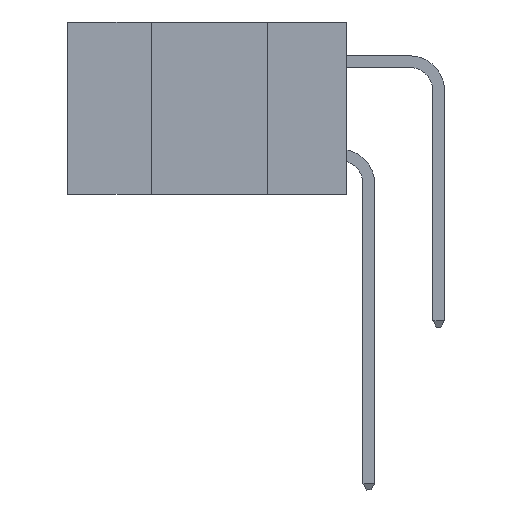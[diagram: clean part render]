
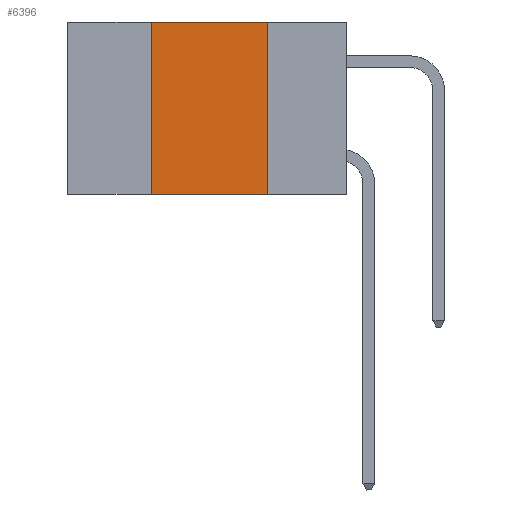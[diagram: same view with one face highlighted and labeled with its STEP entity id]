
A CAD part, left-side view. The second image highlights one B-rep face of the part: STEP entity #6396.
In plain terms, the highlighted planar face has unit normal (-1, 0, 0).
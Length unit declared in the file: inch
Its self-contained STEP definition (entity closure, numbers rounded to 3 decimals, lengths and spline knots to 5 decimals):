
#652 = CARTESIAN_POINT ( 'NONE',  ( 0., 0.6, 0. ) ) ;
#796 = FACE_OUTER_BOUND ( 'NONE', #9455, .T. ) ;
#989 = DIRECTION ( 'NONE',  ( 0., -1., 0. ) ) ;
#1155 = DIRECTION ( 'NONE',  ( 0., -1., 0. ) ) ;
#1907 = CARTESIAN_POINT ( 'NONE',  ( 0., 0.42, -0.37 ) ) ;
#1945 = PLANE ( 'NONE',  #3980 ) ;
#1975 = CARTESIAN_POINT ( 'NONE',  ( 0., 0.17, 0. ) ) ;
#2570 = VERTEX_POINT ( 'NONE', #6561 ) ;
#3783 = ORIENTED_EDGE ( 'NONE', *, *, #4962, .F. ) ;
#3980 = AXIS2_PLACEMENT_3D ( 'NONE', #652, #8829, #10009 ) ;
#4684 = CARTESIAN_POINT ( 'NONE',  ( 0., 0.6, -0.37 ) ) ;
#4962 = EDGE_CURVE ( 'NONE', #5824, #2570, #10721, .T. ) ;
#5193 = CARTESIAN_POINT ( 'NONE',  ( 0., 0.17, 0. ) ) ;
#5269 = VERTEX_POINT ( 'NONE', #1907 ) ;
#5824 = VERTEX_POINT ( 'NONE', #5193 ) ;
#6228 = CARTESIAN_POINT ( 'NONE',  ( 0., 0.6, 0. ) ) ;
#6235 = DIRECTION ( 'NONE',  ( 0., 0., 1. ) ) ;
#6396 = ADVANCED_FACE ( 'NONE', ( #796 ), #1945, .F. ) ;
#6407 = VECTOR ( 'NONE', #1155, 39.37008 ) ;
#6561 = CARTESIAN_POINT ( 'NONE',  ( 0., 0.17, -0.37 ) ) ;
#7607 = VECTOR ( 'NONE', #9014, 39.37008 ) ;
#8057 = EDGE_CURVE ( 'NONE', #5269, #13634, #14396, .T. ) ;
#8186 = ORIENTED_EDGE ( 'NONE', *, *, #12865, .F. ) ;
#8273 = VECTOR ( 'NONE', #989, 39.37008 ) ;
#8553 = ORIENTED_EDGE ( 'NONE', *, *, #14263, .T. ) ;
#8829 = DIRECTION ( 'NONE',  ( 1., 0., 0. ) ) ;
#9014 = DIRECTION ( 'NONE',  ( 0., 0., -1. ) ) ;
#9455 = EDGE_LOOP ( 'NONE', ( #3783, #8186, #11365, #8553 ) ) ;
#9542 = CARTESIAN_POINT ( 'NONE',  ( 0., 0.42, 0. ) ) ;
#9704 = CARTESIAN_POINT ( 'NONE',  ( 0., 0.42, 0. ) ) ;
#10009 = DIRECTION ( 'NONE',  ( 0., 0., -1. ) ) ;
#10259 = LINE ( 'NONE', #4684, #6407 ) ;
#10721 = LINE ( 'NONE', #1975, #7607 ) ;
#11186 = VECTOR ( 'NONE', #6235, 39.37008 ) ;
#11365 = ORIENTED_EDGE ( 'NONE', *, *, #8057, .F. ) ;
#12865 = EDGE_CURVE ( 'NONE', #13634, #5824, #14624, .T. ) ;
#13634 = VERTEX_POINT ( 'NONE', #9542 ) ;
#14263 = EDGE_CURVE ( 'NONE', #5269, #2570, #10259, .T. ) ;
#14396 = LINE ( 'NONE', #9704, #11186 ) ;
#14624 = LINE ( 'NONE', #6228, #8273 ) ;
